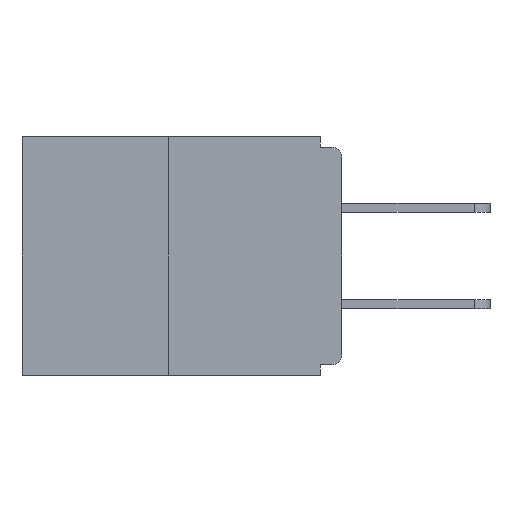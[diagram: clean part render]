
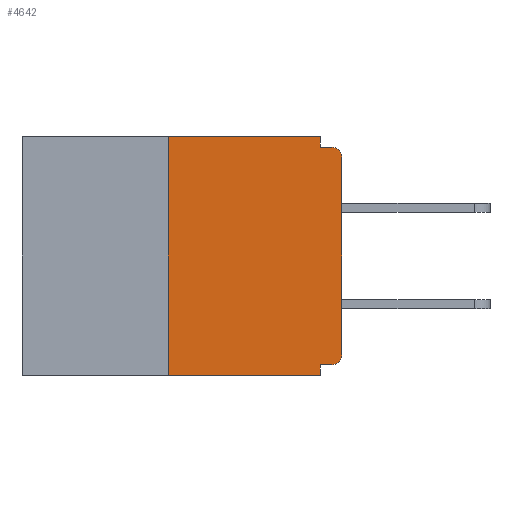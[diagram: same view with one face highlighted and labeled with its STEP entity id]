
A CAD part, left-side view. The second image highlights one B-rep face of the part: STEP entity #4642.
In plain terms, the highlighted planar face has unit normal (-1, 0, 0).
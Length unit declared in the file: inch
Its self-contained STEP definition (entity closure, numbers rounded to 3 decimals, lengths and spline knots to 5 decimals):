
#33 = CIRCLE ( 'NONE', #2027, 0.015 ) ;
#529 = VECTOR ( 'NONE', #3220, 39.37008 ) ;
#731 = DIRECTION ( 'NONE',  ( 0., 0., -1. ) ) ;
#754 = DIRECTION ( 'NONE',  ( -1., 0., 0. ) ) ;
#1412 = LINE ( 'NONE', #10990, #2941 ) ;
#1623 = CARTESIAN_POINT ( 'NONE',  ( 0., 0.015, -0.328 ) ) ;
#1923 = AXIS2_PLACEMENT_3D ( 'NONE', #19967, #15105, #731 ) ;
#2027 = AXIS2_PLACEMENT_3D ( 'NONE', #13617, #754, #15407 ) ;
#2278 = CARTESIAN_POINT ( 'NONE',  ( 0., 0.46, -0.343 ) ) ;
#2492 = CARTESIAN_POINT ( 'NONE',  ( 0., 0., -0.313 ) ) ;
#2830 = VERTEX_POINT ( 'NONE', #2492 ) ;
#2941 = VECTOR ( 'NONE', #7871, 39.37008 ) ;
#3220 = DIRECTION ( 'NONE',  ( 0., -1., 0. ) ) ;
#3224 = EDGE_CURVE ( 'NONE', #7026, #16108, #11607, .T. ) ;
#3293 = EDGE_CURVE ( 'NONE', #9746, #6154, #33, .T. ) ;
#3340 = EDGE_LOOP ( 'NONE', ( #15902, #6479, #15159, #18219, #8414, #11645, #16799, #7166, #14611, #8023 ) ) ;
#3865 = CARTESIAN_POINT ( 'NONE',  ( 0., 0.031, -0.015 ) ) ;
#3892 = CARTESIAN_POINT ( 'NONE',  ( 0., 0.25, 0. ) ) ;
#4089 = DIRECTION ( 'NONE',  ( 1., 0., 0. ) ) ;
#4432 = VECTOR ( 'NONE', #6258, 39.37008 ) ;
#4642 = ADVANCED_FACE ( 'NONE', ( #16169 ), #10275, .F. ) ;
#5114 = VECTOR ( 'NONE', #8709, 39.37008 ) ;
#6083 = CARTESIAN_POINT ( 'NONE',  ( 0., 0.031, 0. ) ) ;
#6154 = VERTEX_POINT ( 'NONE', #13690 ) ;
#6178 = CARTESIAN_POINT ( 'NONE',  ( 0., 0.25, -0.343 ) ) ;
#6258 = DIRECTION ( 'NONE',  ( 0., 0., -1. ) ) ;
#6466 = DIRECTION ( 'NONE',  ( 0., -1., 0. ) ) ;
#6479 = ORIENTED_EDGE ( 'NONE', *, *, #17947, .F. ) ;
#6492 = EDGE_CURVE ( 'NONE', #7026, #2830, #13107, .T. ) ;
#6681 = VERTEX_POINT ( 'NONE', #6083 ) ;
#7026 = VERTEX_POINT ( 'NONE', #1623 ) ;
#7031 = DIRECTION ( 'NONE',  ( 0., 1., 0. ) ) ;
#7166 = ORIENTED_EDGE ( 'NONE', *, *, #3293, .T. ) ;
#7169 = CARTESIAN_POINT ( 'NONE',  ( 0., 0.031, 0. ) ) ;
#7736 = EDGE_CURVE ( 'NONE', #2830, #9746, #18558, .T. ) ;
#7738 = CARTESIAN_POINT ( 'NONE',  ( 0., 0.031, -0.343 ) ) ;
#7871 = DIRECTION ( 'NONE',  ( 0., 0., 1. ) ) ;
#8023 = ORIENTED_EDGE ( 'NONE', *, *, #20380, .F. ) ;
#8089 = CARTESIAN_POINT ( 'NONE',  ( 0., 0., -0.015 ) ) ;
#8276 = VERTEX_POINT ( 'NONE', #3892 ) ;
#8392 = AXIS2_PLACEMENT_3D ( 'NONE', #10414, #4089, #15289 ) ;
#8414 = ORIENTED_EDGE ( 'NONE', *, *, #3224, .F. ) ;
#8709 = DIRECTION ( 'NONE',  ( 0., -1., 0. ) ) ;
#9606 = LINE ( 'NONE', #8089, #529 ) ;
#9746 = VERTEX_POINT ( 'NONE', #19093 ) ;
#10244 = EDGE_CURVE ( 'NONE', #16108, #18435, #14466, .T. ) ;
#10275 = PLANE ( 'NONE',  #8392 ) ;
#10414 = CARTESIAN_POINT ( 'NONE',  ( 0., 0.46, 0. ) ) ;
#10976 = CARTESIAN_POINT ( 'NONE',  ( 0., 0., 0. ) ) ;
#10990 = CARTESIAN_POINT ( 'NONE',  ( 0., 0.25, 0. ) ) ;
#11065 = VECTOR ( 'NONE', #6466, 39.37008 ) ;
#11138 = VECTOR ( 'NONE', #18380, 39.37008 ) ;
#11607 = LINE ( 'NONE', #13418, #16121 ) ;
#11645 = ORIENTED_EDGE ( 'NONE', *, *, #6492, .T. ) ;
#11865 = EDGE_CURVE ( 'NONE', #8276, #6681, #19361, .T. ) ;
#12060 = VERTEX_POINT ( 'NONE', #3865 ) ;
#12657 = LINE ( 'NONE', #7169, #11138 ) ;
#12985 = CARTESIAN_POINT ( 'NONE',  ( 0., 0.46, 0. ) ) ;
#13107 = CIRCLE ( 'NONE', #1923, 0.015 ) ;
#13418 = CARTESIAN_POINT ( 'NONE',  ( 0., 0., -0.328 ) ) ;
#13617 = CARTESIAN_POINT ( 'NONE',  ( 0., 0.015, -0.03 ) ) ;
#13690 = CARTESIAN_POINT ( 'NONE',  ( 0., 0.015, -0.015 ) ) ;
#14466 = LINE ( 'NONE', #7738, #4432 ) ;
#14611 = ORIENTED_EDGE ( 'NONE', *, *, #15959, .F. ) ;
#14641 = VERTEX_POINT ( 'NONE', #6178 ) ;
#15105 = DIRECTION ( 'NONE',  ( -1., 0., 0. ) ) ;
#15159 = ORIENTED_EDGE ( 'NONE', *, *, #15403, .T. ) ;
#15289 = DIRECTION ( 'NONE',  ( 0., 0., -1. ) ) ;
#15403 = EDGE_CURVE ( 'NONE', #14641, #18435, #19422, .T. ) ;
#15407 = DIRECTION ( 'NONE',  ( 0., 0., -1. ) ) ;
#15902 = ORIENTED_EDGE ( 'NONE', *, *, #11865, .F. ) ;
#15959 = EDGE_CURVE ( 'NONE', #12060, #6154, #9606, .T. ) ;
#16108 = VERTEX_POINT ( 'NONE', #19625 ) ;
#16121 = VECTOR ( 'NONE', #7031, 39.37008 ) ;
#16169 = FACE_OUTER_BOUND ( 'NONE', #3340, .T. ) ;
#16799 = ORIENTED_EDGE ( 'NONE', *, *, #7736, .T. ) ;
#17540 = VECTOR ( 'NONE', #18979, 39.37008 ) ;
#17947 = EDGE_CURVE ( 'NONE', #14641, #8276, #1412, .T. ) ;
#18219 = ORIENTED_EDGE ( 'NONE', *, *, #10244, .F. ) ;
#18380 = DIRECTION ( 'NONE',  ( 0., 0., -1. ) ) ;
#18435 = VERTEX_POINT ( 'NONE', #18559 ) ;
#18558 = LINE ( 'NONE', #10976, #17540 ) ;
#18559 = CARTESIAN_POINT ( 'NONE',  ( 0., 0.031, -0.343 ) ) ;
#18979 = DIRECTION ( 'NONE',  ( 0., 0., 1. ) ) ;
#19093 = CARTESIAN_POINT ( 'NONE',  ( 0., 0., -0.03 ) ) ;
#19361 = LINE ( 'NONE', #12985, #11065 ) ;
#19422 = LINE ( 'NONE', #2278, #5114 ) ;
#19625 = CARTESIAN_POINT ( 'NONE',  ( 0., 0.031, -0.328 ) ) ;
#19967 = CARTESIAN_POINT ( 'NONE',  ( 0., 0.015, -0.313 ) ) ;
#20380 = EDGE_CURVE ( 'NONE', #6681, #12060, #12657, .T. ) ;
